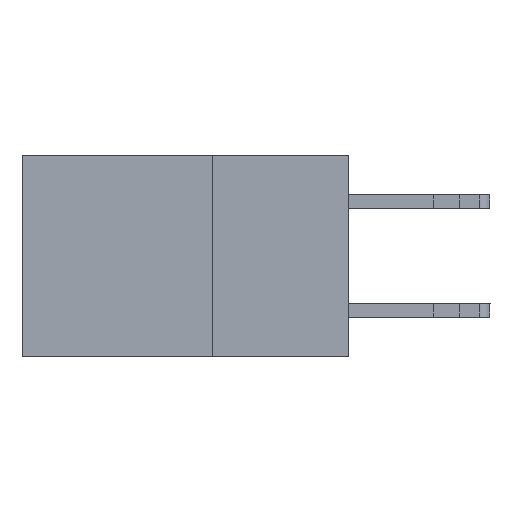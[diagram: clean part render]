
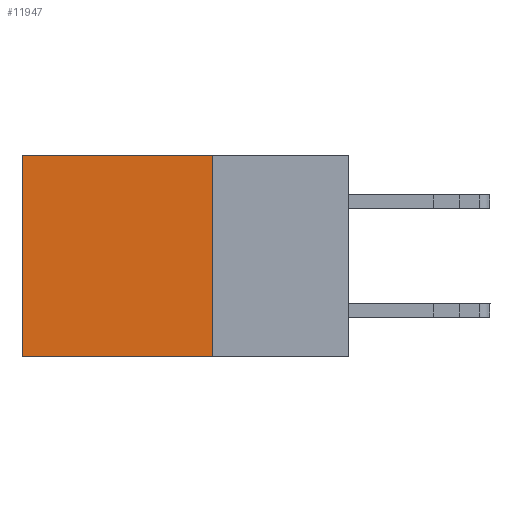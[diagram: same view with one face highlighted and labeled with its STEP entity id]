
A CAD part, left-side view. The second image highlights one B-rep face of the part: STEP entity #11947.
In plain terms, the highlighted planar face has unit normal (-1, 0, 0).
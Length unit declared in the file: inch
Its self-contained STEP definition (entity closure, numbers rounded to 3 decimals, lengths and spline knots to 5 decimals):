
#432 = EDGE_CURVE ( 'NONE', #4869, #14146, #2242, .T. ) ;
#724 = CARTESIAN_POINT ( 'NONE',  ( 0.2615, 0.25, -0.37 ) ) ;
#2020 = ORIENTED_EDGE ( 'NONE', *, *, #8099, .F. ) ;
#2101 = CARTESIAN_POINT ( 'NONE',  ( 0.2615, 0.25, 0. ) ) ;
#2242 = LINE ( 'NONE', #12754, #11733 ) ;
#2278 = DIRECTION ( 'NONE',  ( 0., 0., -1. ) ) ;
#2821 = CARTESIAN_POINT ( 'NONE',  ( 0.2615, 0.6, 0. ) ) ;
#3803 = ORIENTED_EDGE ( 'NONE', *, *, #432, .F. ) ;
#4464 = PLANE ( 'NONE',  #5938 ) ;
#4869 = VERTEX_POINT ( 'NONE', #13356 ) ;
#4936 = ORIENTED_EDGE ( 'NONE', *, *, #13381, .T. ) ;
#5526 = VERTEX_POINT ( 'NONE', #2821 ) ;
#5865 = EDGE_LOOP ( 'NONE', ( #4936, #2020, #3803, #15284 ) ) ;
#5938 = AXIS2_PLACEMENT_3D ( 'NONE', #724, #13826, #6813 ) ;
#6023 = LINE ( 'NONE', #7029, #11942 ) ;
#6408 = VECTOR ( 'NONE', #9200, 39.37008 ) ;
#6813 = DIRECTION ( 'NONE',  ( 0., 0., -1. ) ) ;
#7029 = CARTESIAN_POINT ( 'NONE',  ( 0.2615, 0.6, -0.37 ) ) ;
#7077 = EDGE_CURVE ( 'NONE', #4869, #5526, #11965, .T. ) ;
#7822 = CARTESIAN_POINT ( 'NONE',  ( 0.2615, 0.25, -0.37 ) ) ;
#8099 = EDGE_CURVE ( 'NONE', #14146, #8753, #14189, .T. ) ;
#8753 = VERTEX_POINT ( 'NONE', #11042 ) ;
#9200 = DIRECTION ( 'NONE',  ( 0., 1., 0. ) ) ;
#9983 = DIRECTION ( 'NONE',  ( 0., 1., 0. ) ) ;
#11042 = CARTESIAN_POINT ( 'NONE',  ( 0.2615, 0.6, -0.37 ) ) ;
#11116 = CARTESIAN_POINT ( 'NONE',  ( 0.2615, 0.25, -0.37 ) ) ;
#11123 = VECTOR ( 'NONE', #9983, 39.37008 ) ;
#11266 = DIRECTION ( 'NONE',  ( 0., 0., -1. ) ) ;
#11733 = VECTOR ( 'NONE', #11266, 39.37008 ) ;
#11942 = VECTOR ( 'NONE', #2278, 39.37008 ) ;
#11947 = ADVANCED_FACE ( 'NONE', ( #13398 ), #4464, .F. ) ;
#11965 = LINE ( 'NONE', #2101, #6408 ) ;
#12754 = CARTESIAN_POINT ( 'NONE',  ( 0.2615, 0.25, -0.37 ) ) ;
#13356 = CARTESIAN_POINT ( 'NONE',  ( 0.2615, 0.25, 0. ) ) ;
#13381 = EDGE_CURVE ( 'NONE', #5526, #8753, #6023, .T. ) ;
#13398 = FACE_OUTER_BOUND ( 'NONE', #5865, .T. ) ;
#13826 = DIRECTION ( 'NONE',  ( 1., 0., 0. ) ) ;
#14146 = VERTEX_POINT ( 'NONE', #7822 ) ;
#14189 = LINE ( 'NONE', #11116, #11123 ) ;
#15284 = ORIENTED_EDGE ( 'NONE', *, *, #7077, .T. ) ;
